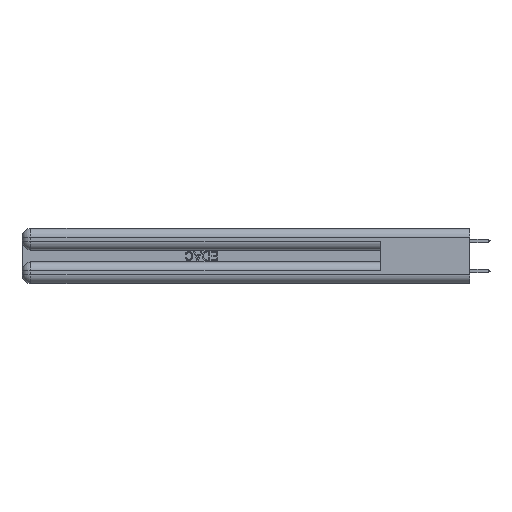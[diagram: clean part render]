
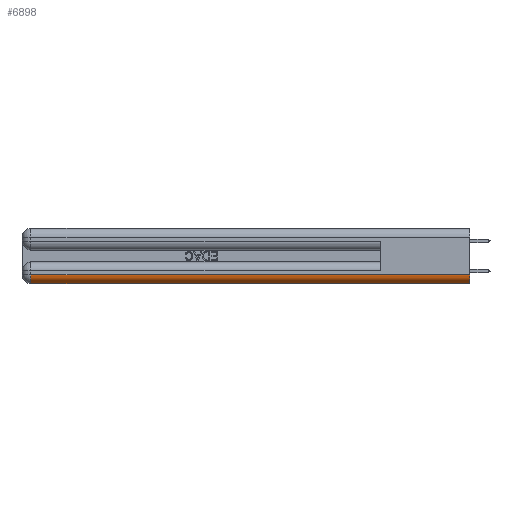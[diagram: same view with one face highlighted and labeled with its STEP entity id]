
A CAD part, left-side view. The second image highlights one B-rep face of the part: STEP entity #6898.
In plain terms, the highlighted cylindrical face has radius 1.524 mm (diameter 3.048 mm), a partial arc.
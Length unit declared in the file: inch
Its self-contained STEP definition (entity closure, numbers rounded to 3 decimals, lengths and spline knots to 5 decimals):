
#3818 = ORIENTED_EDGE ( 'NONE', *, *, #34779, .F. ) ;
#4124 = EDGE_CURVE ( 'NONE', #29034, #4691, #13652, .T. ) ;
#4691 = VERTEX_POINT ( 'NONE', #18680 ) ;
#4701 = VECTOR ( 'NONE', #25443, 39.37008 ) ;
#4958 = FACE_OUTER_BOUND ( 'NONE', #27492, .T. ) ;
#5473 = VERTEX_POINT ( 'NONE', #29755 ) ;
#6328 = CARTESIAN_POINT ( 'NONE',  ( 0.06, 0., 0.06 ) ) ;
#6898 = ADVANCED_FACE ( 'NONE', ( #4958 ), #21770, .T. ) ;
#7119 = CARTESIAN_POINT ( 'NONE',  ( 0.06, 2.94, 0.06 ) ) ;
#9134 = EDGE_CURVE ( 'NONE', #4691, #39756, #27225, .T. ) ;
#9309 = VECTOR ( 'NONE', #13385, 39.37008 ) ;
#10507 = DIRECTION ( 'NONE',  ( 0., 0., 1. ) ) ;
#11859 = CARTESIAN_POINT ( 'NONE',  ( 0., 2.94, 0.06 ) ) ;
#13385 = DIRECTION ( 'NONE',  ( 0., -1., 0. ) ) ;
#13652 = LINE ( 'NONE', #25299, #4701 ) ;
#14129 = AXIS2_PLACEMENT_3D ( 'NONE', #35818, #15703, #39127 ) ;
#14403 = CARTESIAN_POINT ( 'NONE',  ( 0.06, 0., 0. ) ) ;
#15703 = DIRECTION ( 'NONE',  ( 0., -1., 0. ) ) ;
#16440 = DIRECTION ( 'NONE',  ( 0., 0., 1. ) ) ;
#17013 = ORIENTED_EDGE ( 'NONE', *, *, #23536, .F. ) ;
#18680 = CARTESIAN_POINT ( 'NONE',  ( 0.06, 2.94, 0. ) ) ;
#19266 = LINE ( 'NONE', #26711, #9309 ) ;
#21770 = CYLINDRICAL_SURFACE ( 'NONE', #31089, 0.06 ) ;
#23065 = ORIENTED_EDGE ( 'NONE', *, *, #4124, .F. ) ;
#23536 = EDGE_CURVE ( 'NONE', #39756, #5473, #19266, .T. ) ;
#24466 = ORIENTED_EDGE ( 'NONE', *, *, #9134, .F. ) ;
#25299 = CARTESIAN_POINT ( 'NONE',  ( 0.06, 3., 0. ) ) ;
#25443 = DIRECTION ( 'NONE',  ( 0., 1., 0. ) ) ;
#26711 = CARTESIAN_POINT ( 'NONE',  ( 0., 0., 0.06 ) ) ;
#27178 = CIRCLE ( 'NONE', #14129, 0.06 ) ;
#27225 = CIRCLE ( 'NONE', #41711, 0.06 ) ;
#27492 = EDGE_LOOP ( 'NONE', ( #3818, #17013, #24466, #23065 ) ) ;
#29034 = VERTEX_POINT ( 'NONE', #14403 ) ;
#29755 = CARTESIAN_POINT ( 'NONE',  ( 0., 0., 0.06 ) ) ;
#30582 = DIRECTION ( 'NONE',  ( 0., 1., 0. ) ) ;
#31089 = AXIS2_PLACEMENT_3D ( 'NONE', #6328, #36543, #16440 ) ;
#34779 = EDGE_CURVE ( 'NONE', #5473, #29034, #27178, .T. ) ;
#35818 = CARTESIAN_POINT ( 'NONE',  ( 0.06, 0., 0.06 ) ) ;
#36543 = DIRECTION ( 'NONE',  ( 0., 1., 0. ) ) ;
#39127 = DIRECTION ( 'NONE',  ( 0., 0., 1. ) ) ;
#39756 = VERTEX_POINT ( 'NONE', #11859 ) ;
#41711 = AXIS2_PLACEMENT_3D ( 'NONE', #7119, #30582, #10507 ) ;
